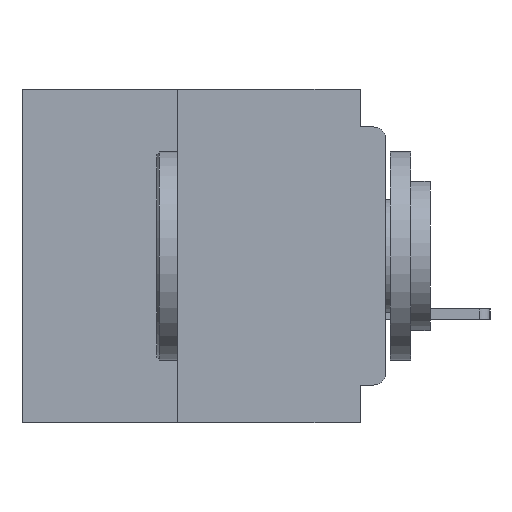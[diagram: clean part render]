
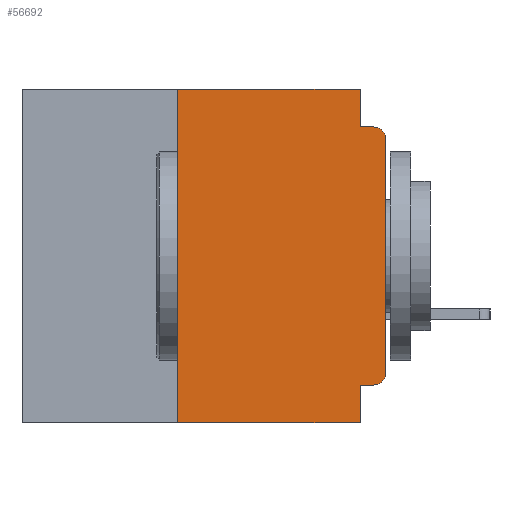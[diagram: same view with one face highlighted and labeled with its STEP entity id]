
A CAD part, left-side view. The second image highlights one B-rep face of the part: STEP entity #56692.
In plain terms, the highlighted planar face has unit normal (-1, 0, 0).
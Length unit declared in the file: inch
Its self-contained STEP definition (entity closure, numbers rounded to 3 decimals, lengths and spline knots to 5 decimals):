
#85 = DIRECTION ( 'NONE',  ( 1., 0., 0. ) ) ;
#407 = CARTESIAN_POINT ( 'NONE',  ( 0., 0.015, -0.34 ) ) ;
#1579 = CARTESIAN_POINT ( 'NONE',  ( 0., 0., -0.045 ) ) ;
#1993 = EDGE_CURVE ( 'NONE', #26789, #50686, #38030, .T. ) ;
#2161 = EDGE_CURVE ( 'NONE', #36120, #5400, #52943, .T. ) ;
#2892 = LINE ( 'NONE', #18239, #26823 ) ;
#3375 = ORIENTED_EDGE ( 'NONE', *, *, #6024, .T. ) ;
#3562 = VECTOR ( 'NONE', #12419, 39.37008 ) ;
#3815 = DIRECTION ( 'NONE',  ( 0., -1., 0. ) ) ;
#4079 = VERTEX_POINT ( 'NONE', #21357 ) ;
#5200 = DIRECTION ( 'NONE',  ( 0., 0., -1. ) ) ;
#5400 = VERTEX_POINT ( 'NONE', #6280 ) ;
#5885 = EDGE_CURVE ( 'NONE', #42697, #61123, #48047, .T. ) ;
#6024 = EDGE_CURVE ( 'NONE', #61123, #39895, #26326, .T. ) ;
#6213 = CARTESIAN_POINT ( 'NONE',  ( 0., 0., 0. ) ) ;
#6280 = CARTESIAN_POINT ( 'NONE',  ( 0., 0.031, -0.4 ) ) ;
#6956 = EDGE_CURVE ( 'NONE', #30914, #59649, #2892, .T. ) ;
#8043 = EDGE_CURVE ( 'NONE', #39895, #50686, #38642, .T. ) ;
#8355 = CARTESIAN_POINT ( 'NONE',  ( 0., 0.031, 0. ) ) ;
#8386 = DIRECTION ( 'NONE',  ( 0., 0., -1. ) ) ;
#8592 = CARTESIAN_POINT ( 'NONE',  ( 0., 0.031, 0. ) ) ;
#12419 = DIRECTION ( 'NONE',  ( 0., -1., 0. ) ) ;
#12508 = CARTESIAN_POINT ( 'NONE',  ( 0., 0.015, -0.355 ) ) ;
#12563 = VECTOR ( 'NONE', #35048, 39.37008 ) ;
#12724 = EDGE_CURVE ( 'NONE', #59649, #26789, #52260, .T. ) ;
#14106 = VECTOR ( 'NONE', #8386, 39.37008 ) ;
#14436 = EDGE_CURVE ( 'NONE', #36120, #30914, #17721, .T. ) ;
#14969 = ORIENTED_EDGE ( 'NONE', *, *, #1993, .F. ) ;
#16105 = ORIENTED_EDGE ( 'NONE', *, *, #25932, .F. ) ;
#16296 = CARTESIAN_POINT ( 'NONE',  ( 0., 0., -0.06 ) ) ;
#17515 = CARTESIAN_POINT ( 'NONE',  ( 0., 0.25, 0. ) ) ;
#17721 = LINE ( 'NONE', #59786, #48382 ) ;
#18239 = CARTESIAN_POINT ( 'NONE',  ( 0., 0.437, 0. ) ) ;
#19692 = LINE ( 'NONE', #35255, #43620 ) ;
#21357 = CARTESIAN_POINT ( 'NONE',  ( 0., 0.031, -0.355 ) ) ;
#23323 = CARTESIAN_POINT ( 'NONE',  ( 0., 0.015, -0.06 ) ) ;
#23920 = CARTESIAN_POINT ( 'NONE',  ( 0., 0.437, 0. ) ) ;
#25437 = CARTESIAN_POINT ( 'NONE',  ( 0., 0.031, -0.4 ) ) ;
#25458 = DIRECTION ( 'NONE',  ( 0., 0., 1. ) ) ;
#25618 = DIRECTION ( 'NONE',  ( 0., 1., 0. ) ) ;
#25932 = EDGE_CURVE ( 'NONE', #42697, #4079, #19692, .T. ) ;
#26304 = ORIENTED_EDGE ( 'NONE', *, *, #5885, .T. ) ;
#26326 = LINE ( 'NONE', #6213, #50259 ) ;
#26537 = DIRECTION ( 'NONE',  ( 0., 0., 1. ) ) ;
#26789 = VERTEX_POINT ( 'NONE', #61095 ) ;
#26823 = VECTOR ( 'NONE', #3815, 39.37008 ) ;
#28188 = DIRECTION ( 'NONE',  ( 0., 0., -1. ) ) ;
#29415 = AXIS2_PLACEMENT_3D ( 'NONE', #407, #33867, #5200 ) ;
#29568 = EDGE_CURVE ( 'NONE', #4079, #5400, #58962, .T. ) ;
#30253 = ORIENTED_EDGE ( 'NONE', *, *, #12724, .F. ) ;
#30914 = VERTEX_POINT ( 'NONE', #17515 ) ;
#31584 = ORIENTED_EDGE ( 'NONE', *, *, #29568, .F. ) ;
#31675 = CARTESIAN_POINT ( 'NONE',  ( 0., 0.437, -0.4 ) ) ;
#33542 = VECTOR ( 'NONE', #35076, 39.37008 ) ;
#33556 = DIRECTION ( 'NONE',  ( 0., 0., -1. ) ) ;
#33867 = DIRECTION ( 'NONE',  ( -1., 0., 0. ) ) ;
#35048 = DIRECTION ( 'NONE',  ( 0., -1., 0. ) ) ;
#35076 = DIRECTION ( 'NONE',  ( 0., 0., -1. ) ) ;
#35255 = CARTESIAN_POINT ( 'NONE',  ( 0., 0., -0.355 ) ) ;
#36120 = VERTEX_POINT ( 'NONE', #56083 ) ;
#38030 = LINE ( 'NONE', #1579, #12563 ) ;
#38642 = CIRCLE ( 'NONE', #43471, 0.015 ) ;
#39895 = VERTEX_POINT ( 'NONE', #16296 ) ;
#42697 = VERTEX_POINT ( 'NONE', #12508 ) ;
#43047 = EDGE_LOOP ( 'NONE', ( #3375, #49546, #14969, #30253, #47727, #56887, #49955, #31584, #16105, #26304 ) ) ;
#43471 = AXIS2_PLACEMENT_3D ( 'NONE', #23323, #56808, #28188 ) ;
#43620 = VECTOR ( 'NONE', #25618, 39.37008 ) ;
#47727 = ORIENTED_EDGE ( 'NONE', *, *, #6956, .F. ) ;
#48047 = CIRCLE ( 'NONE', #29415, 0.015 ) ;
#48357 = CARTESIAN_POINT ( 'NONE',  ( 0., 0., -0.34 ) ) ;
#48382 = VECTOR ( 'NONE', #26537, 39.37008 ) ;
#49093 = CARTESIAN_POINT ( 'NONE',  ( 0., 0.015, -0.045 ) ) ;
#49546 = ORIENTED_EDGE ( 'NONE', *, *, #8043, .T. ) ;
#49955 = ORIENTED_EDGE ( 'NONE', *, *, #2161, .T. ) ;
#50259 = VECTOR ( 'NONE', #25458, 39.37008 ) ;
#50686 = VERTEX_POINT ( 'NONE', #49093 ) ;
#52260 = LINE ( 'NONE', #8592, #14106 ) ;
#52546 = PLANE ( 'NONE',  #57306 ) ;
#52943 = LINE ( 'NONE', #31675, #3562 ) ;
#56083 = CARTESIAN_POINT ( 'NONE',  ( 0., 0.25, -0.4 ) ) ;
#56692 = ADVANCED_FACE ( 'NONE', ( #58291 ), #52546, .F. ) ;
#56808 = DIRECTION ( 'NONE',  ( -1., 0., 0. ) ) ;
#56887 = ORIENTED_EDGE ( 'NONE', *, *, #14436, .F. ) ;
#57306 = AXIS2_PLACEMENT_3D ( 'NONE', #23920, #85, #33556 ) ;
#58291 = FACE_OUTER_BOUND ( 'NONE', #43047, .T. ) ;
#58962 = LINE ( 'NONE', #25437, #33542 ) ;
#59649 = VERTEX_POINT ( 'NONE', #8355 ) ;
#59786 = CARTESIAN_POINT ( 'NONE',  ( 0., 0.25, -0.4 ) ) ;
#61095 = CARTESIAN_POINT ( 'NONE',  ( 0., 0.031, -0.045 ) ) ;
#61123 = VERTEX_POINT ( 'NONE', #48357 ) ;
